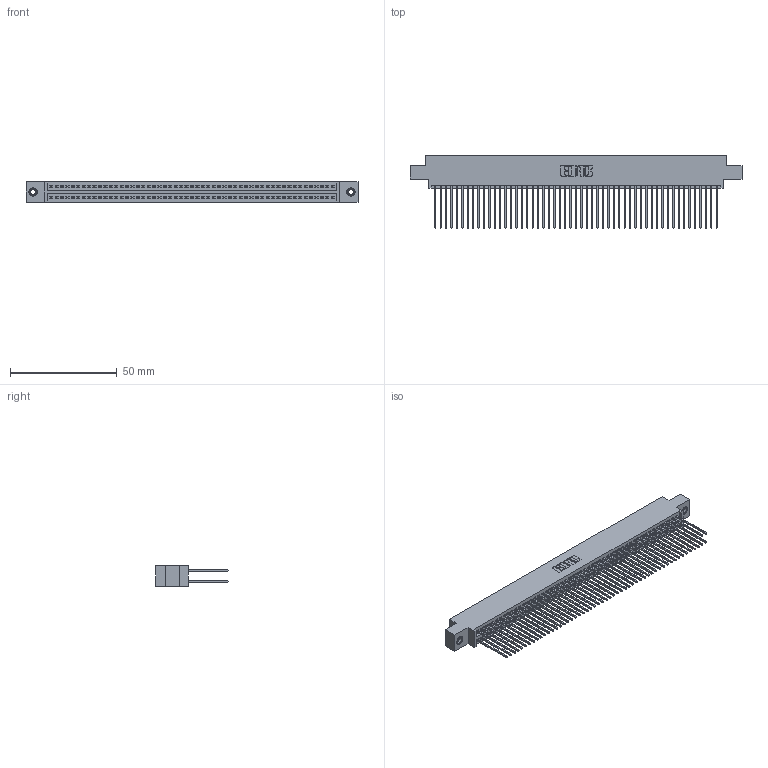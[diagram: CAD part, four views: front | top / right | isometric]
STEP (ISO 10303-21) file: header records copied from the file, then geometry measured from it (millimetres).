
FILE_DESCRIPTION (( 'STEP AP203' ), '1' );
FILE_NAME ('395-106-541-808.STEP', '2019-10-27T05:20:13', ( '' ), ( '' ), 'SwSTEP 2.0', 'SolidWorks 2016', '' );
FILE_SCHEMA (( 'CONFIG_CONTROL_DESIGN' ));
Length unit declared in the file: inch
Products named in the file (4): 345 Part_0.170 Offset - 0.156 Dia-TI; 345-292-001_345-293-141; 345-250-001_345-250-003-102; 395-106-541-808
Assembly tree (109 placements, depth 2):
  395-106-541-808
    345 Part_0.170 Offset - 0.156 Dia-TI
    345-292-001_345-293-141  x106
    345-250-001_345-250-003-102  x2
Bounding box: 155.83 x 33.96 x 9.4 mm (x, y, z)
Volume: 15727.7 mm3; surface area: 26476.9 mm2
Topology: 109 solids, 109 shells, 5490 faces, 16283 edges, 10706 vertices
Faces by surface type: plane 3614, cylinder 1860, cone 12, torus 4
Entity records: 41440 total; most frequent: CARTESIAN_POINT 6919, ORIENTED_EDGE 6846, DIRECTION 6113, EDGE_CURVE 3423, LINE 3059, VECTOR 3059, VERTEX_POINT 2276, AXIS2_PLACEMENT_3D 1527
